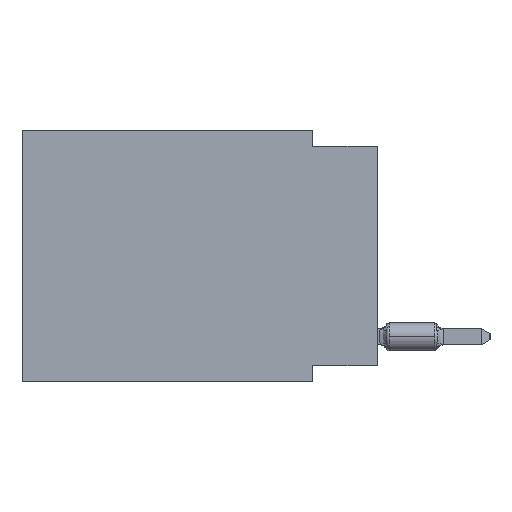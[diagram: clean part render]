
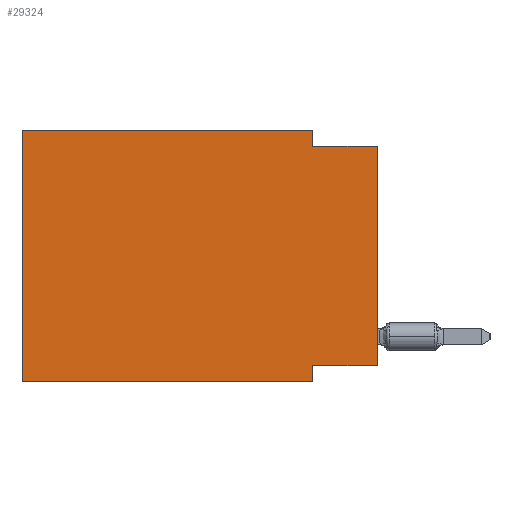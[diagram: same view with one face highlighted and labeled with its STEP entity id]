
A CAD part, left-side view. The second image highlights one B-rep face of the part: STEP entity #29324.
In plain terms, the highlighted planar face has unit normal (-1, 0, 0).
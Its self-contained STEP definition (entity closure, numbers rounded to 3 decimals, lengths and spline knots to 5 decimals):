
#1941 = FACE_OUTER_BOUND ( 'NONE', #22886, .T. ) ;
#2325 = DIRECTION ( 'NONE',  ( 1., 0., 0. ) ) ;
#2505 = CARTESIAN_POINT ( 'NONE',  ( 0., 0.55, -0.39 ) ) ;
#4338 = VERTEX_POINT ( 'NONE', #37244 ) ;
#7494 = LINE ( 'NONE', #31727, #58544 ) ;
#7528 = VECTOR ( 'NONE', #76718, 39.37008 ) ;
#7792 = VECTOR ( 'NONE', #12742, 39.37008 ) ;
#8062 = EDGE_CURVE ( 'NONE', #46504, #4338, #25865, .T. ) ;
#8661 = PLANE ( 'NONE',  #35107 ) ;
#9335 = CARTESIAN_POINT ( 'NONE',  ( 0., 0., -0.025 ) ) ;
#10440 = LINE ( 'NONE', #22326, #17815 ) ;
#10794 = VECTOR ( 'NONE', #67933, 39.37008 ) ;
#11178 = CARTESIAN_POINT ( 'NONE',  ( 0., 0., -0.365 ) ) ;
#11595 = DIRECTION ( 'NONE',  ( 0., 1., 0. ) ) ;
#11737 = EDGE_CURVE ( 'NONE', #42690, #24141, #31379, .T. ) ;
#11785 = CARTESIAN_POINT ( 'NONE',  ( 0., 0.1, -0.365 ) ) ;
#12742 = DIRECTION ( 'NONE',  ( 0., 0., -1. ) ) ;
#14926 = VECTOR ( 'NONE', #11595, 39.37008 ) ;
#15664 = CARTESIAN_POINT ( 'NONE',  ( 0., 0.1, -0.025 ) ) ;
#16475 = LINE ( 'NONE', #76844, #62283 ) ;
#17006 = ORIENTED_EDGE ( 'NONE', *, *, #52624, .F. ) ;
#17314 = ORIENTED_EDGE ( 'NONE', *, *, #28154, .F. ) ;
#17815 = VECTOR ( 'NONE', #41369, 39.37008 ) ;
#20930 = VERTEX_POINT ( 'NONE', #15664 ) ;
#22326 = CARTESIAN_POINT ( 'NONE',  ( 0., 0., -0.025 ) ) ;
#22886 = EDGE_LOOP ( 'NONE', ( #61891, #27076, #17314, #37237, #17006, #47046, #38358, #34118 ) ) ;
#24141 = VERTEX_POINT ( 'NONE', #9335 ) ;
#25041 = LINE ( 'NONE', #49268, #7792 ) ;
#25865 = LINE ( 'NONE', #27049, #10794 ) ;
#27049 = CARTESIAN_POINT ( 'NONE',  ( 0., 0.1, -0.39 ) ) ;
#27076 = ORIENTED_EDGE ( 'NONE', *, *, #34039, .F. ) ;
#27888 = VECTOR ( 'NONE', #42116, 39.37008 ) ;
#28154 = EDGE_CURVE ( 'NONE', #34284, #20930, #25041, .T. ) ;
#29324 = ADVANCED_FACE ( 'NONE', ( #1941 ), #8661, .F. ) ;
#30439 = EDGE_CURVE ( 'NONE', #42690, #46504, #47350, .T. ) ;
#30658 = CARTESIAN_POINT ( 'NONE',  ( 0., 0.55, -0.39 ) ) ;
#31379 = LINE ( 'NONE', #73468, #27888 ) ;
#31727 = CARTESIAN_POINT ( 'NONE',  ( 0., 0.55, 0. ) ) ;
#32896 = DIRECTION ( 'NONE',  ( 0., 0., -1. ) ) ;
#34039 = EDGE_CURVE ( 'NONE', #20930, #24141, #10440, .T. ) ;
#34118 = ORIENTED_EDGE ( 'NONE', *, *, #30439, .F. ) ;
#34284 = VERTEX_POINT ( 'NONE', #62449 ) ;
#35107 = AXIS2_PLACEMENT_3D ( 'NONE', #63493, #2325, #32896 ) ;
#37095 = VERTEX_POINT ( 'NONE', #51216 ) ;
#37237 = ORIENTED_EDGE ( 'NONE', *, *, #69211, .F. ) ;
#37244 = CARTESIAN_POINT ( 'NONE',  ( 0., 0.1, -0.39 ) ) ;
#38358 = ORIENTED_EDGE ( 'NONE', *, *, #8062, .F. ) ;
#41369 = DIRECTION ( 'NONE',  ( 0., -1., 0. ) ) ;
#41881 = DIRECTION ( 'NONE',  ( 0., 0., 1. ) ) ;
#42116 = DIRECTION ( 'NONE',  ( 0., 0., 1. ) ) ;
#42690 = VERTEX_POINT ( 'NONE', #74603 ) ;
#46504 = VERTEX_POINT ( 'NONE', #11785 ) ;
#47046 = ORIENTED_EDGE ( 'NONE', *, *, #77366, .T. ) ;
#47325 = VERTEX_POINT ( 'NONE', #30658 ) ;
#47350 = LINE ( 'NONE', #11178, #14926 ) ;
#49268 = CARTESIAN_POINT ( 'NONE',  ( 0., 0.1, 0. ) ) ;
#51216 = CARTESIAN_POINT ( 'NONE',  ( 0., 0.55, 0. ) ) ;
#52624 = EDGE_CURVE ( 'NONE', #47325, #37095, #16475, .T. ) ;
#56722 = DIRECTION ( 'NONE',  ( 0., -1., 0. ) ) ;
#58544 = VECTOR ( 'NONE', #56722, 39.37008 ) ;
#61891 = ORIENTED_EDGE ( 'NONE', *, *, #11737, .T. ) ;
#62283 = VECTOR ( 'NONE', #41881, 39.37008 ) ;
#62449 = CARTESIAN_POINT ( 'NONE',  ( 0., 0.1, 0. ) ) ;
#63493 = CARTESIAN_POINT ( 'NONE',  ( 0., 0.55, 0. ) ) ;
#67933 = DIRECTION ( 'NONE',  ( 0., 0., -1. ) ) ;
#69211 = EDGE_CURVE ( 'NONE', #37095, #34284, #7494, .T. ) ;
#73468 = CARTESIAN_POINT ( 'NONE',  ( 0., 0., 0. ) ) ;
#74603 = CARTESIAN_POINT ( 'NONE',  ( 0., 0., -0.365 ) ) ;
#75953 = LINE ( 'NONE', #2505, #7528 ) ;
#76718 = DIRECTION ( 'NONE',  ( 0., -1., 0. ) ) ;
#76844 = CARTESIAN_POINT ( 'NONE',  ( 0., 0.55, 0. ) ) ;
#77366 = EDGE_CURVE ( 'NONE', #47325, #4338, #75953, .T. ) ;
